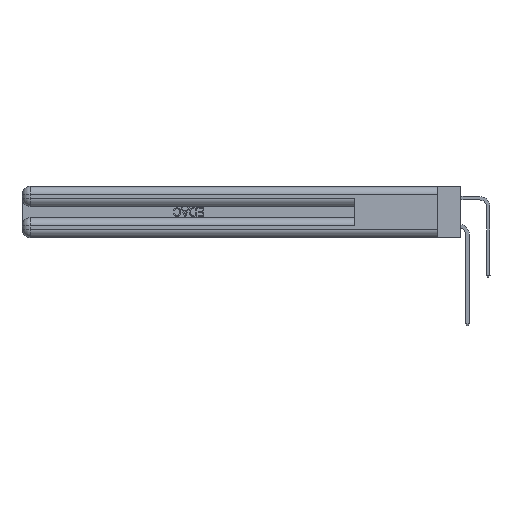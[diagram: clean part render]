
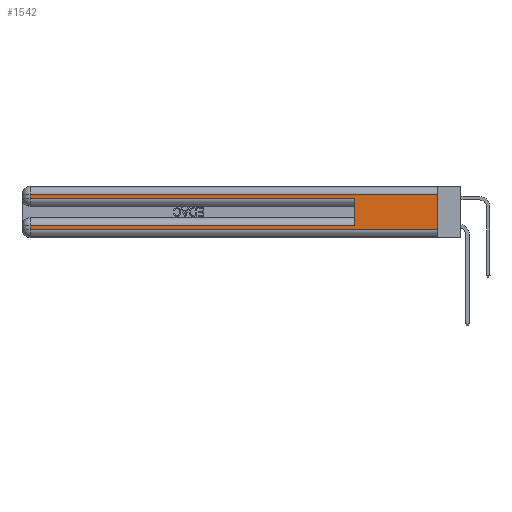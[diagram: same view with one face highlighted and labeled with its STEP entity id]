
A CAD part, left-side view. The second image highlights one B-rep face of the part: STEP entity #1542.
In plain terms, the highlighted planar face has unit normal (-1, 0, 0).
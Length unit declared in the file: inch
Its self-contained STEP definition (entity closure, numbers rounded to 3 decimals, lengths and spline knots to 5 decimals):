
#362 = CARTESIAN_POINT ( 'NONE',  ( 0., 2.94, 0.37 ) ) ;
#1295 = DIRECTION ( 'NONE',  ( 0., 1., 0. ) ) ;
#1542 = ADVANCED_FACE ( 'NONE', ( #29601 ), #8126, .F. ) ;
#2942 = CARTESIAN_POINT ( 'NONE',  ( 0., 0., 0.37 ) ) ;
#4878 = ORIENTED_EDGE ( 'NONE', *, *, #26033, .F. ) ;
#4967 = VECTOR ( 'NONE', #15397, 39.37008 ) ;
#5321 = CARTESIAN_POINT ( 'NONE',  ( 0., 2.94, 0.285 ) ) ;
#5601 = DIRECTION ( 'NONE',  ( 0., 0., -1. ) ) ;
#5912 = LINE ( 'NONE', #10551, #41263 ) ;
#7006 = EDGE_CURVE ( 'NONE', #8470, #13724, #37996, .T. ) ;
#7124 = DIRECTION ( 'NONE',  ( 0., -1., 0. ) ) ;
#7198 = CARTESIAN_POINT ( 'NONE',  ( 0., 0., 0.085 ) ) ;
#7642 = ORIENTED_EDGE ( 'NONE', *, *, #14547, .F. ) ;
#8126 = PLANE ( 'NONE',  #19895 ) ;
#8470 = VERTEX_POINT ( 'NONE', #23182 ) ;
#9855 = ORIENTED_EDGE ( 'NONE', *, *, #44823, .T. ) ;
#10465 = VECTOR ( 'NONE', #38389, 39.37008 ) ;
#10551 = CARTESIAN_POINT ( 'NONE',  ( 0., 0., 0.285 ) ) ;
#10960 = LINE ( 'NONE', #7198, #38007 ) ;
#11801 = CARTESIAN_POINT ( 'NONE',  ( 0., 0.6, 0.145 ) ) ;
#11939 = CARTESIAN_POINT ( 'NONE',  ( 0., 0., 0.31 ) ) ;
#13164 = LINE ( 'NONE', #24517, #21516 ) ;
#13724 = VERTEX_POINT ( 'NONE', #39018 ) ;
#14126 = VECTOR ( 'NONE', #5601, 39.37008 ) ;
#14547 = EDGE_CURVE ( 'NONE', #16277, #24180, #15607, .T. ) ;
#15303 = CARTESIAN_POINT ( 'NONE',  ( 0., 0., 0.37 ) ) ;
#15397 = DIRECTION ( 'NONE',  ( 0., 0., 1. ) ) ;
#15607 = LINE ( 'NONE', #11801, #4967 ) ;
#16277 = VERTEX_POINT ( 'NONE', #31290 ) ;
#16390 = EDGE_CURVE ( 'NONE', #22047, #24180, #5912, .T. ) ;
#17480 = LINE ( 'NONE', #23355, #14126 ) ;
#18880 = DIRECTION ( 'NONE',  ( 0., 0., -1. ) ) ;
#19895 = AXIS2_PLACEMENT_3D ( 'NONE', #15303, #39895, #18880 ) ;
#19964 = EDGE_CURVE ( 'NONE', #29011, #42841, #43442, .T. ) ;
#21039 = LINE ( 'NONE', #2942, #10465 ) ;
#21516 = VECTOR ( 'NONE', #45468, 39.37008 ) ;
#21763 = DIRECTION ( 'NONE',  ( 0., 0., -1. ) ) ;
#22047 = VERTEX_POINT ( 'NONE', #5321 ) ;
#22635 = EDGE_CURVE ( 'NONE', #42841, #22047, #17480, .T. ) ;
#22812 = CARTESIAN_POINT ( 'NONE',  ( 0., 0., 0.06 ) ) ;
#23182 = CARTESIAN_POINT ( 'NONE',  ( 0., 2.94, 0.085 ) ) ;
#23355 = CARTESIAN_POINT ( 'NONE',  ( 0., 2.94, 0.37 ) ) ;
#23841 = ORIENTED_EDGE ( 'NONE', *, *, #19964, .T. ) ;
#24180 = VERTEX_POINT ( 'NONE', #45403 ) ;
#24517 = CARTESIAN_POINT ( 'NONE',  ( 0., 0., 0.06 ) ) ;
#26033 = EDGE_CURVE ( 'NONE', #29011, #39994, #21039, .T. ) ;
#26332 = EDGE_LOOP ( 'NONE', ( #4878, #23841, #33147, #34726, #7642, #9855, #28761, #40215 ) ) ;
#27844 = EDGE_CURVE ( 'NONE', #13724, #39994, #13164, .T. ) ;
#28478 = CARTESIAN_POINT ( 'NONE',  ( 0., 2.94, 0.31 ) ) ;
#28484 = DIRECTION ( 'NONE',  ( 0., 1., 0. ) ) ;
#28761 = ORIENTED_EDGE ( 'NONE', *, *, #7006, .T. ) ;
#29011 = VERTEX_POINT ( 'NONE', #41089 ) ;
#29601 = FACE_OUTER_BOUND ( 'NONE', #26332, .T. ) ;
#31290 = CARTESIAN_POINT ( 'NONE',  ( 0., 0.6, 0.085 ) ) ;
#33147 = ORIENTED_EDGE ( 'NONE', *, *, #22635, .T. ) ;
#34123 = VECTOR ( 'NONE', #1295, 39.37008 ) ;
#34726 = ORIENTED_EDGE ( 'NONE', *, *, #16390, .T. ) ;
#36886 = VECTOR ( 'NONE', #21763, 39.37008 ) ;
#37996 = LINE ( 'NONE', #362, #36886 ) ;
#38007 = VECTOR ( 'NONE', #28484, 39.37008 ) ;
#38389 = DIRECTION ( 'NONE',  ( 0., 0., -1. ) ) ;
#39018 = CARTESIAN_POINT ( 'NONE',  ( 0., 2.94, 0.06 ) ) ;
#39895 = DIRECTION ( 'NONE',  ( 1., 0., 0. ) ) ;
#39994 = VERTEX_POINT ( 'NONE', #22812 ) ;
#40215 = ORIENTED_EDGE ( 'NONE', *, *, #27844, .T. ) ;
#41089 = CARTESIAN_POINT ( 'NONE',  ( 0., 0., 0.31 ) ) ;
#41263 = VECTOR ( 'NONE', #7124, 39.37008 ) ;
#42841 = VERTEX_POINT ( 'NONE', #28478 ) ;
#43442 = LINE ( 'NONE', #11939, #34123 ) ;
#44823 = EDGE_CURVE ( 'NONE', #16277, #8470, #10960, .T. ) ;
#45403 = CARTESIAN_POINT ( 'NONE',  ( 0., 0.6, 0.285 ) ) ;
#45468 = DIRECTION ( 'NONE',  ( 0., -1., 0. ) ) ;
